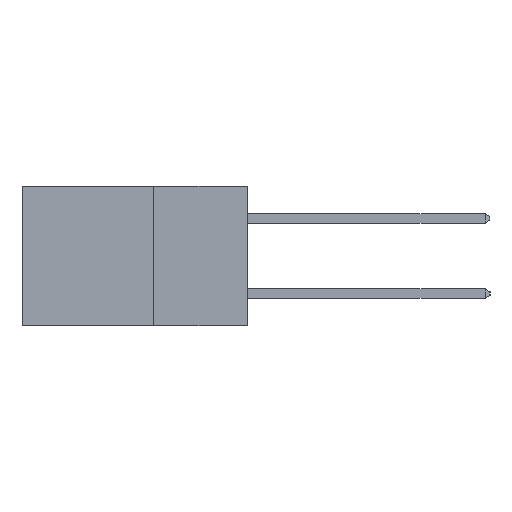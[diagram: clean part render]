
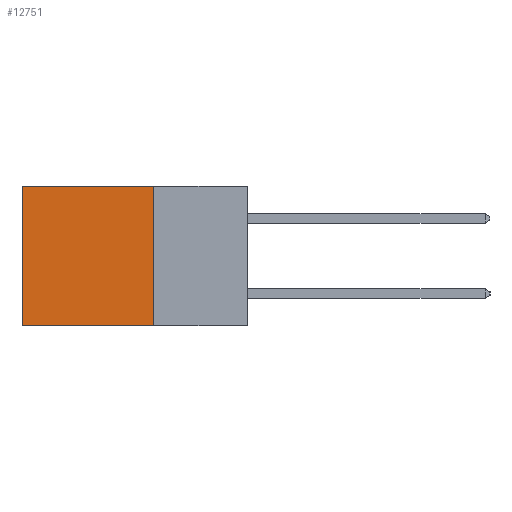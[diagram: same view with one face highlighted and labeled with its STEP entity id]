
A CAD part, left-side view. The second image highlights one B-rep face of the part: STEP entity #12751.
In plain terms, the highlighted planar face has unit normal (-1, 0, 0).
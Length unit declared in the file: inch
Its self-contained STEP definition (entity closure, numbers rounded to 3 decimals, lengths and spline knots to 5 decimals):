
#159 = FACE_OUTER_BOUND ( 'NONE', #11758, .T. ) ;
#376 = DIRECTION ( 'NONE',  ( 0., 0., -1. ) ) ;
#1291 = DIRECTION ( 'NONE',  ( 0., 1., 0. ) ) ;
#1525 = VERTEX_POINT ( 'NONE', #13435 ) ;
#2598 = CARTESIAN_POINT ( 'NONE',  ( 0.2615, 0.25, -0.37 ) ) ;
#3649 = AXIS2_PLACEMENT_3D ( 'NONE', #2598, #12901, #4077 ) ;
#4012 = PLANE ( 'NONE',  #3649 ) ;
#4027 = LINE ( 'NONE', #8683, #7536 ) ;
#4077 = DIRECTION ( 'NONE',  ( 0., 0., -1. ) ) ;
#4391 = EDGE_CURVE ( 'NONE', #13418, #9749, #4027, .T. ) ;
#4489 = CARTESIAN_POINT ( 'NONE',  ( 0.2615, 0.6, -0.37 ) ) ;
#4684 = CARTESIAN_POINT ( 'NONE',  ( 0.2615, 0.25, 0. ) ) ;
#5315 = EDGE_CURVE ( 'NONE', #1525, #9749, #11379, .T. ) ;
#6276 = CARTESIAN_POINT ( 'NONE',  ( 0.2615, 0.25, -0.37 ) ) ;
#7451 = LINE ( 'NONE', #6276, #11335 ) ;
#7497 = VECTOR ( 'NONE', #17801, 39.37008 ) ;
#7536 = VECTOR ( 'NONE', #1291, 39.37008 ) ;
#7713 = ORIENTED_EDGE ( 'NONE', *, *, #5315, .T. ) ;
#7843 = VECTOR ( 'NONE', #16596, 39.37008 ) ;
#8076 = EDGE_CURVE ( 'NONE', #15403, #1525, #11744, .T. ) ;
#8683 = CARTESIAN_POINT ( 'NONE',  ( 0.2615, 0.25, -0.37 ) ) ;
#9749 = VERTEX_POINT ( 'NONE', #4489 ) ;
#10748 = ORIENTED_EDGE ( 'NONE', *, *, #8076, .T. ) ;
#10773 = EDGE_CURVE ( 'NONE', #15403, #13418, #7451, .T. ) ;
#11335 = VECTOR ( 'NONE', #376, 39.37008 ) ;
#11379 = LINE ( 'NONE', #16349, #7497 ) ;
#11744 = LINE ( 'NONE', #17547, #7843 ) ;
#11758 = EDGE_LOOP ( 'NONE', ( #7713, #15674, #18007, #10748 ) ) ;
#12751 = ADVANCED_FACE ( 'NONE', ( #159 ), #4012, .F. ) ;
#12901 = DIRECTION ( 'NONE',  ( 1., 0., 0. ) ) ;
#13418 = VERTEX_POINT ( 'NONE', #14524 ) ;
#13435 = CARTESIAN_POINT ( 'NONE',  ( 0.2615, 0.6, 0. ) ) ;
#14524 = CARTESIAN_POINT ( 'NONE',  ( 0.2615, 0.25, -0.37 ) ) ;
#15403 = VERTEX_POINT ( 'NONE', #4684 ) ;
#15674 = ORIENTED_EDGE ( 'NONE', *, *, #4391, .F. ) ;
#16349 = CARTESIAN_POINT ( 'NONE',  ( 0.2615, 0.6, -0.37 ) ) ;
#16596 = DIRECTION ( 'NONE',  ( 0., 1., 0. ) ) ;
#17547 = CARTESIAN_POINT ( 'NONE',  ( 0.2615, 0.25, 0. ) ) ;
#17801 = DIRECTION ( 'NONE',  ( 0., 0., -1. ) ) ;
#18007 = ORIENTED_EDGE ( 'NONE', *, *, #10773, .F. ) ;
